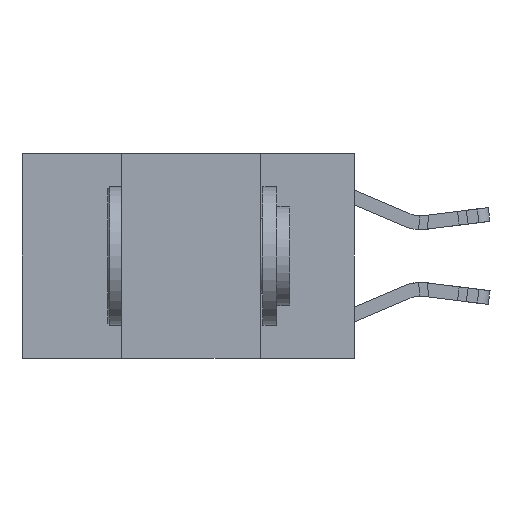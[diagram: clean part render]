
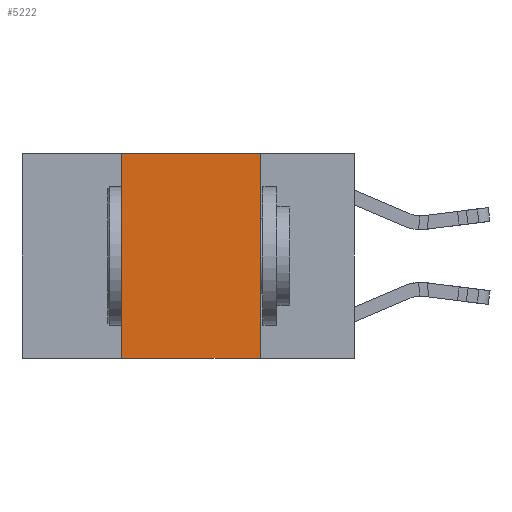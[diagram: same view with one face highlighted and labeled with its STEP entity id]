
A CAD part, left-side view. The second image highlights one B-rep face of the part: STEP entity #5222.
In plain terms, the highlighted planar face has unit normal (-1, 0, 0).
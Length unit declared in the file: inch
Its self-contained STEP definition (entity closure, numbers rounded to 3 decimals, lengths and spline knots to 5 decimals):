
#337 = FACE_OUTER_BOUND ( 'NONE', #25394, .T. ) ;
#2676 = VECTOR ( 'NONE', #16439, 39.37008 ) ;
#2692 = VECTOR ( 'NONE', #15012, 39.37008 ) ;
#3840 = CARTESIAN_POINT ( 'NONE',  ( 0., 0.42, 0. ) ) ;
#5222 = ADVANCED_FACE ( 'NONE', ( #337 ), #20076, .F. ) ;
#5223 = ORIENTED_EDGE ( 'NONE', *, *, #10563, .T. ) ;
#8344 = LINE ( 'NONE', #3840, #13882 ) ;
#9749 = EDGE_CURVE ( 'NONE', #30515, #13612, #8344, .T. ) ;
#10188 = EDGE_CURVE ( 'NONE', #29934, #24382, #14602, .T. ) ;
#10563 = EDGE_CURVE ( 'NONE', #30515, #24382, #11470, .T. ) ;
#10671 = DIRECTION ( 'NONE',  ( 1., 0., 0. ) ) ;
#11470 = LINE ( 'NONE', #25600, #23307 ) ;
#12329 = CARTESIAN_POINT ( 'NONE',  ( 0., 0.17, 0. ) ) ;
#13612 = VERTEX_POINT ( 'NONE', #19093 ) ;
#13882 = VECTOR ( 'NONE', #25146, 39.37008 ) ;
#14602 = LINE ( 'NONE', #26763, #2692 ) ;
#14768 = EDGE_CURVE ( 'NONE', #13612, #29934, #21621, .T. ) ;
#14870 = ORIENTED_EDGE ( 'NONE', *, *, #10188, .F. ) ;
#15012 = DIRECTION ( 'NONE',  ( 0., 0., -1. ) ) ;
#16439 = DIRECTION ( 'NONE',  ( 0., -1., 0. ) ) ;
#18484 = DIRECTION ( 'NONE',  ( 0., -1., 0. ) ) ;
#18789 = AXIS2_PLACEMENT_3D ( 'NONE', #29408, #10671, #27173 ) ;
#19093 = CARTESIAN_POINT ( 'NONE',  ( 0., 0.42, 0. ) ) ;
#19114 = CARTESIAN_POINT ( 'NONE',  ( 0., 0.42, -0.37 ) ) ;
#20076 = PLANE ( 'NONE',  #18789 ) ;
#21158 = ORIENTED_EDGE ( 'NONE', *, *, #14768, .F. ) ;
#21621 = LINE ( 'NONE', #25823, #2676 ) ;
#22652 = ORIENTED_EDGE ( 'NONE', *, *, #9749, .F. ) ;
#23307 = VECTOR ( 'NONE', #18484, 39.37008 ) ;
#24382 = VERTEX_POINT ( 'NONE', #28017 ) ;
#25146 = DIRECTION ( 'NONE',  ( 0., 0., 1. ) ) ;
#25394 = EDGE_LOOP ( 'NONE', ( #14870, #21158, #22652, #5223 ) ) ;
#25600 = CARTESIAN_POINT ( 'NONE',  ( 0., 0.6, -0.37 ) ) ;
#25823 = CARTESIAN_POINT ( 'NONE',  ( 0., 0.6, 0. ) ) ;
#26763 = CARTESIAN_POINT ( 'NONE',  ( 0., 0.17, 0. ) ) ;
#27173 = DIRECTION ( 'NONE',  ( 0., 0., -1. ) ) ;
#28017 = CARTESIAN_POINT ( 'NONE',  ( 0., 0.17, -0.37 ) ) ;
#29408 = CARTESIAN_POINT ( 'NONE',  ( 0., 0.6, 0. ) ) ;
#29934 = VERTEX_POINT ( 'NONE', #12329 ) ;
#30515 = VERTEX_POINT ( 'NONE', #19114 ) ;
